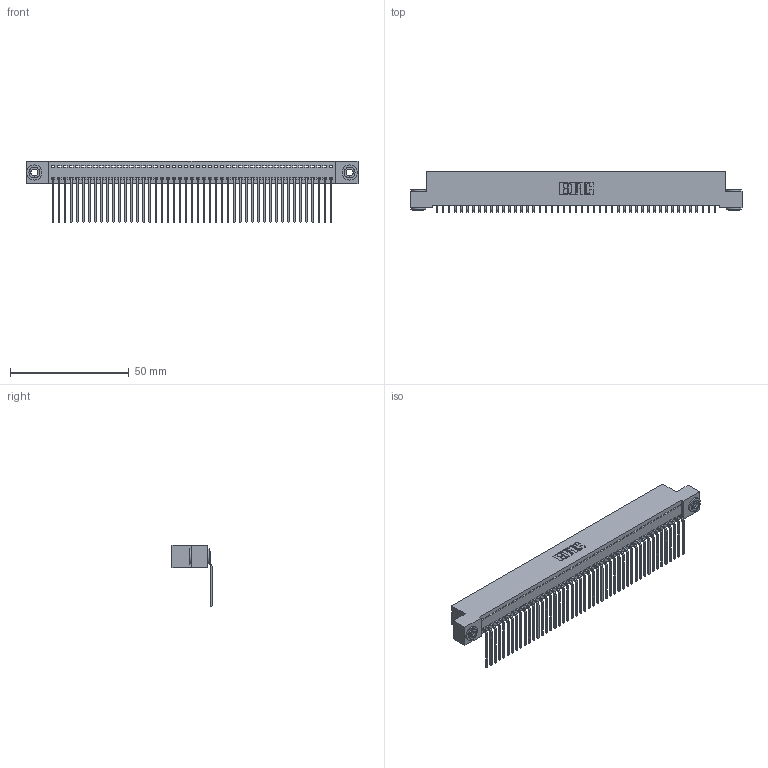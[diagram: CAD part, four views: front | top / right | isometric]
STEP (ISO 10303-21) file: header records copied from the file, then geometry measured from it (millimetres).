
FILE_DESCRIPTION (( 'STEP AP203' ), '1' );
FILE_NAME ('392-047-559-103.STEP', '2018-08-16T21:25:49', ( '' ), ( '' ), 'SwSTEP 2.0', 'SolidWorks 2016', '' );
FILE_SCHEMA (( 'CONFIG_CONTROL_DESIGN' ));
Length unit declared in the file: inch
Products named in the file (4): 342 Part_.156 TH; 345-292-001_558 559 Tail - 1; 342-250-002_345-250-002-102; 392-047-559-103
Assembly tree (50 placements, depth 2):
  392-047-559-103
    342 Part_.156 TH
    345-292-001_558 559 Tail - 1  x47
    342-250-002_345-250-002-102  x2
Bounding box: 139.7 x 16.83 x 25.78 mm (x, y, z)
Volume: 12446.7 mm3; surface area: 19486.3 mm2
Topology: 50 solids, 50 shells, 2968 faces, 8929 edges, 5886 vertices
Faces by surface type: plane 2144, cylinder 816, cone 8
Entity records: 28688 total; most frequent: CARTESIAN_POINT 4926, ORIENTED_EDGE 4902, DIRECTION 4179, EDGE_CURVE 2451, LINE 2299, VECTOR 2299, VERTEX_POINT 1630, AXIS2_PLACEMENT_3D 940
